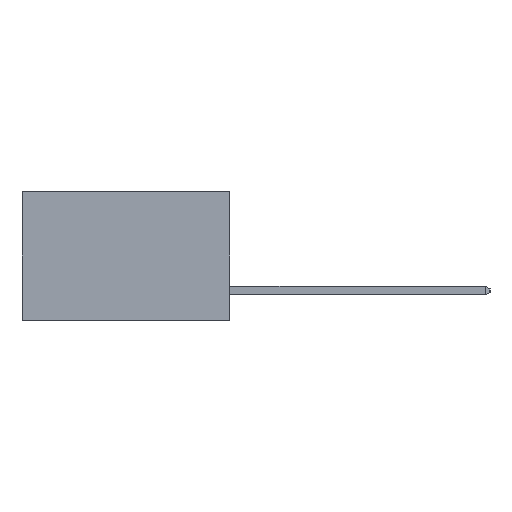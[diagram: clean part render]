
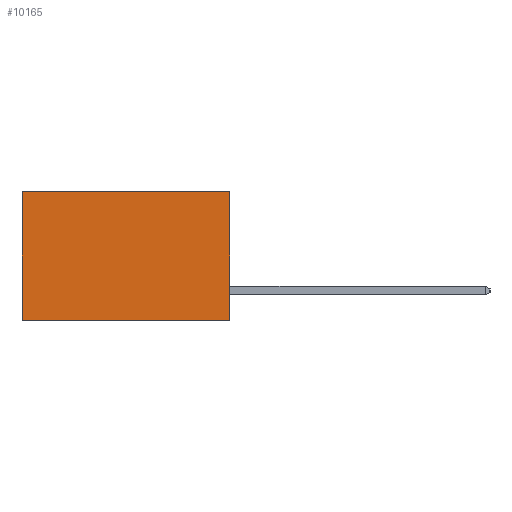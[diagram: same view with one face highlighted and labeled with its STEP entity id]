
A CAD part, left-side view. The second image highlights one B-rep face of the part: STEP entity #10165.
In plain terms, the highlighted planar face has unit normal (-1, 0, 0).
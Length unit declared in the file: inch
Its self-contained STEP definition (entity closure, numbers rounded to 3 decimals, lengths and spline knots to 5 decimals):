
#771 = EDGE_CURVE ( 'NONE', #11006, #15149, #12410, .T. ) ;
#864 = EDGE_CURVE ( 'NONE', #13121, #15149, #12981, .T. ) ;
#912 = EDGE_CURVE ( 'NONE', #1302, #13121, #14322, .T. ) ;
#1302 = VERTEX_POINT ( 'NONE', #8771 ) ;
#1533 = CARTESIAN_POINT ( 'NONE',  ( 0.298, 0., -0.37 ) ) ;
#1922 = DIRECTION ( 'NONE',  ( 1., 0., 0. ) ) ;
#2112 = CARTESIAN_POINT ( 'NONE',  ( 0.298, 0.6, -0.37 ) ) ;
#2406 = CARTESIAN_POINT ( 'NONE',  ( 0.298, 0.6, 0. ) ) ;
#2491 = DIRECTION ( 'NONE',  ( 0., 0., -1. ) ) ;
#2714 = FACE_OUTER_BOUND ( 'NONE', #3466, .T. ) ;
#3105 = VECTOR ( 'NONE', #7569, 39.37008 ) ;
#3113 = ORIENTED_EDGE ( 'NONE', *, *, #771, .T. ) ;
#3415 = CARTESIAN_POINT ( 'NONE',  ( 0.298, 0., 0. ) ) ;
#3466 = EDGE_LOOP ( 'NONE', ( #3113, #13227, #7843, #11540 ) ) ;
#7421 = AXIS2_PLACEMENT_3D ( 'NONE', #9315, #1922, #10589 ) ;
#7569 = DIRECTION ( 'NONE',  ( 0., 1., 0. ) ) ;
#7641 = CARTESIAN_POINT ( 'NONE',  ( 0.298, 0., -0.37 ) ) ;
#7843 = ORIENTED_EDGE ( 'NONE', *, *, #912, .F. ) ;
#8771 = CARTESIAN_POINT ( 'NONE',  ( 0.298, 0., 0. ) ) ;
#9315 = CARTESIAN_POINT ( 'NONE',  ( 0.298, 0., 0. ) ) ;
#9586 = EDGE_CURVE ( 'NONE', #1302, #11006, #15632, .T. ) ;
#10165 = ADVANCED_FACE ( 'NONE', ( #2714 ), #14281, .F. ) ;
#10589 = DIRECTION ( 'NONE',  ( 0., 0., -1. ) ) ;
#10846 = DIRECTION ( 'NONE',  ( 0., 1., 0. ) ) ;
#11006 = VERTEX_POINT ( 'NONE', #2406 ) ;
#11056 = VECTOR ( 'NONE', #11718, 39.37008 ) ;
#11540 = ORIENTED_EDGE ( 'NONE', *, *, #9586, .T. ) ;
#11718 = DIRECTION ( 'NONE',  ( 0., 0., -1. ) ) ;
#12362 = CARTESIAN_POINT ( 'NONE',  ( 0.298, 0., 0. ) ) ;
#12410 = LINE ( 'NONE', #14604, #15263 ) ;
#12981 = LINE ( 'NONE', #1533, #3105 ) ;
#13121 = VERTEX_POINT ( 'NONE', #7641 ) ;
#13227 = ORIENTED_EDGE ( 'NONE', *, *, #864, .F. ) ;
#14281 = PLANE ( 'NONE',  #7421 ) ;
#14322 = LINE ( 'NONE', #12362, #11056 ) ;
#14604 = CARTESIAN_POINT ( 'NONE',  ( 0.298, 0.6, 0. ) ) ;
#15149 = VERTEX_POINT ( 'NONE', #2112 ) ;
#15263 = VECTOR ( 'NONE', #2491, 39.37008 ) ;
#15264 = VECTOR ( 'NONE', #10846, 39.37008 ) ;
#15632 = LINE ( 'NONE', #3415, #15264 ) ;
